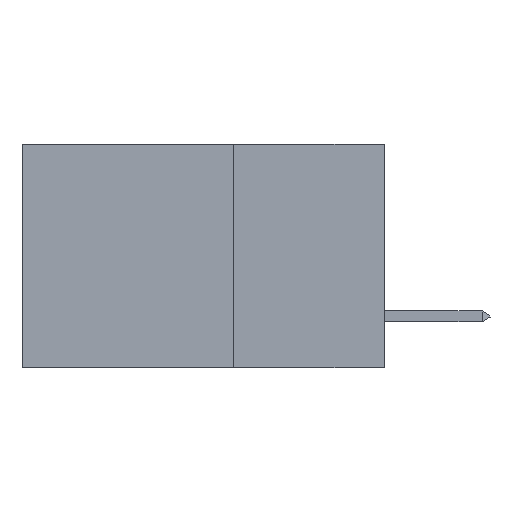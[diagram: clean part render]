
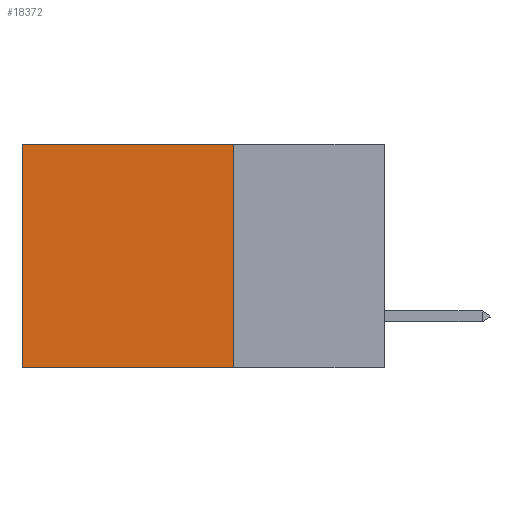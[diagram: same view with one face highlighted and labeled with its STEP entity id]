
A CAD part, left-side view. The second image highlights one B-rep face of the part: STEP entity #18372.
In plain terms, the highlighted planar face has unit normal (-1, 0, 0).
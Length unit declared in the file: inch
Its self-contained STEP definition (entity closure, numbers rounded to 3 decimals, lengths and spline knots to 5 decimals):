
#585 = VECTOR ( 'NONE', #1043, 39.37008 ) ;
#686 = VERTEX_POINT ( 'NONE', #7568 ) ;
#999 = EDGE_LOOP ( 'NONE', ( #14061, #2746, #7369, #14930 ) ) ;
#1043 = DIRECTION ( 'NONE',  ( 0., 1., 0. ) ) ;
#1638 = CARTESIAN_POINT ( 'NONE',  ( 0.2875, 0.25, 0. ) ) ;
#1761 = VERTEX_POINT ( 'NONE', #8646 ) ;
#2746 = ORIENTED_EDGE ( 'NONE', *, *, #12331, .F. ) ;
#3402 = DIRECTION ( 'NONE',  ( 0., 0., -1. ) ) ;
#3606 = LINE ( 'NONE', #13779, #10869 ) ;
#4139 = AXIS2_PLACEMENT_3D ( 'NONE', #12458, #15674, #17168 ) ;
#4423 = CARTESIAN_POINT ( 'NONE',  ( 0.2875, 0.6, 0. ) ) ;
#6406 = EDGE_CURVE ( 'NONE', #13515, #1761, #9114, .T. ) ;
#6417 = LINE ( 'NONE', #17066, #585 ) ;
#7076 = VECTOR ( 'NONE', #11162, 39.37008 ) ;
#7369 = ORIENTED_EDGE ( 'NONE', *, *, #12068, .F. ) ;
#7568 = CARTESIAN_POINT ( 'NONE',  ( 0.2875, 0.25, -0.37 ) ) ;
#8646 = CARTESIAN_POINT ( 'NONE',  ( 0.2875, 0.6, -0.37 ) ) ;
#9114 = LINE ( 'NONE', #15951, #13982 ) ;
#10071 = VERTEX_POINT ( 'NONE', #1638 ) ;
#10869 = VECTOR ( 'NONE', #3402, 39.37008 ) ;
#11162 = DIRECTION ( 'NONE',  ( 0., 1., 0. ) ) ;
#11512 = DIRECTION ( 'NONE',  ( 0., 0., -1. ) ) ;
#12068 = EDGE_CURVE ( 'NONE', #10071, #686, #3606, .T. ) ;
#12316 = CARTESIAN_POINT ( 'NONE',  ( 0.2875, 0.25, 0. ) ) ;
#12331 = EDGE_CURVE ( 'NONE', #686, #1761, #6417, .T. ) ;
#12458 = CARTESIAN_POINT ( 'NONE',  ( 0.2875, 0.25, 0. ) ) ;
#13515 = VERTEX_POINT ( 'NONE', #4423 ) ;
#13779 = CARTESIAN_POINT ( 'NONE',  ( 0.2875, 0.25, 0. ) ) ;
#13982 = VECTOR ( 'NONE', #11512, 39.37008 ) ;
#14061 = ORIENTED_EDGE ( 'NONE', *, *, #6406, .T. ) ;
#14127 = EDGE_CURVE ( 'NONE', #10071, #13515, #15223, .T. ) ;
#14149 = PLANE ( 'NONE',  #4139 ) ;
#14930 = ORIENTED_EDGE ( 'NONE', *, *, #14127, .T. ) ;
#15223 = LINE ( 'NONE', #12316, #7076 ) ;
#15674 = DIRECTION ( 'NONE',  ( 1., 0., 0. ) ) ;
#15951 = CARTESIAN_POINT ( 'NONE',  ( 0.2875, 0.6, 0. ) ) ;
#17066 = CARTESIAN_POINT ( 'NONE',  ( 0.2875, 0.25, -0.37 ) ) ;
#17132 = FACE_OUTER_BOUND ( 'NONE', #999, .T. ) ;
#17168 = DIRECTION ( 'NONE',  ( 0., 0., -1. ) ) ;
#18372 = ADVANCED_FACE ( 'NONE', ( #17132 ), #14149, .F. ) ;
